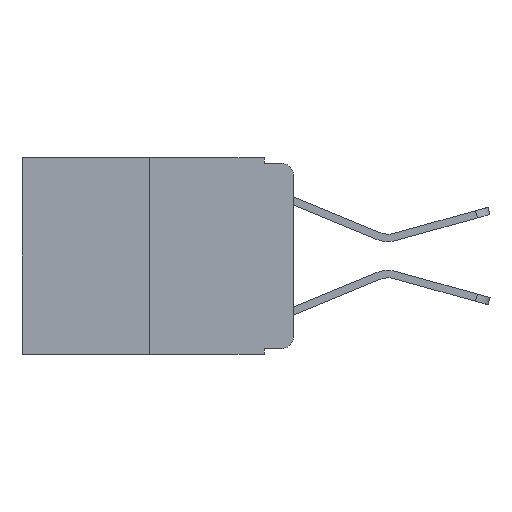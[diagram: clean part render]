
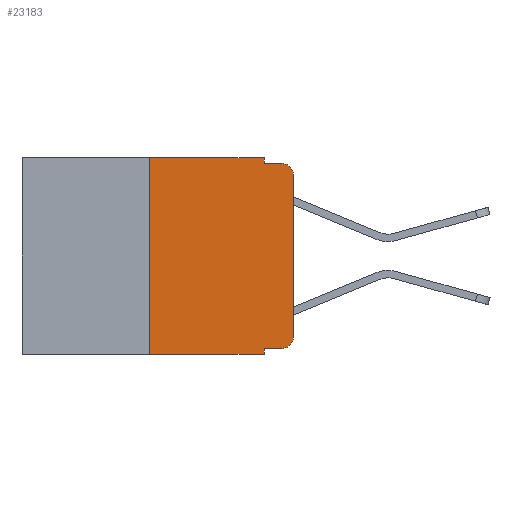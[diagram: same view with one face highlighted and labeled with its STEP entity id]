
A CAD part, left-side view. The second image highlights one B-rep face of the part: STEP entity #23183.
In plain terms, the highlighted planar face has unit normal (-1, 0, 0).
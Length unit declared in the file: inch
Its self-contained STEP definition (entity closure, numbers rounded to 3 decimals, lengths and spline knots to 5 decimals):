
#263 = CARTESIAN_POINT ( 'NONE',  ( 0., 0.473, 0. ) ) ;
#602 = VERTEX_POINT ( 'NONE', #15090 ) ;
#735 = DIRECTION ( 'NONE',  ( 0., 0., -1. ) ) ;
#879 = ORIENTED_EDGE ( 'NONE', *, *, #21196, .T. ) ;
#1485 = CARTESIAN_POINT ( 'NONE',  ( 0., 0.473, -0.343 ) ) ;
#1562 = EDGE_CURVE ( 'NONE', #11115, #17570, #9679, .T. ) ;
#1811 = ORIENTED_EDGE ( 'NONE', *, *, #1562, .T. ) ;
#1951 = ORIENTED_EDGE ( 'NONE', *, *, #12078, .F. ) ;
#2250 = CARTESIAN_POINT ( 'NONE',  ( 0., 0.25, 0. ) ) ;
#3317 = VERTEX_POINT ( 'NONE', #5917 ) ;
#3351 = DIRECTION ( 'NONE',  ( 0., 0., -1. ) ) ;
#3401 = CARTESIAN_POINT ( 'NONE',  ( 0., 0.051, -0.343 ) ) ;
#3549 = EDGE_CURVE ( 'NONE', #8855, #22190, #14930, .T. ) ;
#3611 = CARTESIAN_POINT ( 'NONE',  ( 0., 0., -0.313 ) ) ;
#4162 = CARTESIAN_POINT ( 'NONE',  ( 0., 0.051, -0.01 ) ) ;
#4498 = VECTOR ( 'NONE', #6863, 39.37008 ) ;
#5495 = VERTEX_POINT ( 'NONE', #8070 ) ;
#5668 = DIRECTION ( 'NONE',  ( 0., 0., -1. ) ) ;
#5885 = VERTEX_POINT ( 'NONE', #8922 ) ;
#5917 = CARTESIAN_POINT ( 'NONE',  ( 0., 0.051, -0.333 ) ) ;
#6086 = CARTESIAN_POINT ( 'NONE',  ( 0., 0.02, -0.03 ) ) ;
#6502 = ORIENTED_EDGE ( 'NONE', *, *, #15943, .T. ) ;
#6740 = EDGE_CURVE ( 'NONE', #602, #15473, #20439, .T. ) ;
#6863 = DIRECTION ( 'NONE',  ( 0., 0., 1. ) ) ;
#6919 = VECTOR ( 'NONE', #9512, 39.37008 ) ;
#6938 = VERTEX_POINT ( 'NONE', #21496 ) ;
#8070 = CARTESIAN_POINT ( 'NONE',  ( 0., 0.25, 0. ) ) ;
#8281 = LINE ( 'NONE', #10126, #20691 ) ;
#8409 = ORIENTED_EDGE ( 'NONE', *, *, #22758, .F. ) ;
#8703 = CIRCLE ( 'NONE', #23043, 0.02 ) ;
#8769 = CARTESIAN_POINT ( 'NONE',  ( 0., 0.051, 0. ) ) ;
#8855 = VERTEX_POINT ( 'NONE', #3611 ) ;
#8922 = CARTESIAN_POINT ( 'NONE',  ( 0., 0.02, -0.333 ) ) ;
#9144 = DIRECTION ( 'NONE',  ( 1., 0., 0. ) ) ;
#9228 = EDGE_CURVE ( 'NONE', #5495, #6938, #14072, .T. ) ;
#9345 = ORIENTED_EDGE ( 'NONE', *, *, #3549, .T. ) ;
#9499 = DIRECTION ( 'NONE',  ( 0., 0., 1. ) ) ;
#9512 = DIRECTION ( 'NONE',  ( 0., -1., 0. ) ) ;
#9598 = LINE ( 'NONE', #2250, #11291 ) ;
#9679 = LINE ( 'NONE', #1485, #13357 ) ;
#9899 = DIRECTION ( 'NONE',  ( 0., -1., 0. ) ) ;
#10126 = CARTESIAN_POINT ( 'NONE',  ( 0., 0.051, 0. ) ) ;
#10714 = PLANE ( 'NONE',  #14123 ) ;
#10947 = CARTESIAN_POINT ( 'NONE',  ( 0., 0.25, -0.343 ) ) ;
#11115 = VERTEX_POINT ( 'NONE', #10947 ) ;
#11219 = DIRECTION ( 'NONE',  ( 0., -1., 0. ) ) ;
#11291 = VECTOR ( 'NONE', #9499, 39.37008 ) ;
#11510 = DIRECTION ( 'NONE',  ( -1., 0., 0. ) ) ;
#11651 = CARTESIAN_POINT ( 'NONE',  ( 0., 0.02, -0.01 ) ) ;
#11848 = ORIENTED_EDGE ( 'NONE', *, *, #13816, .F. ) ;
#11943 = DIRECTION ( 'NONE',  ( 0., 0., -1. ) ) ;
#12078 = EDGE_CURVE ( 'NONE', #3317, #17570, #8281, .T. ) ;
#12957 = ORIENTED_EDGE ( 'NONE', *, *, #9228, .F. ) ;
#13031 = LINE ( 'NONE', #16780, #19215 ) ;
#13125 = ORIENTED_EDGE ( 'NONE', *, *, #17053, .T. ) ;
#13357 = VECTOR ( 'NONE', #23028, 39.37008 ) ;
#13458 = LINE ( 'NONE', #8769, #16560 ) ;
#13816 = EDGE_CURVE ( 'NONE', #11115, #5495, #9598, .T. ) ;
#14063 = CIRCLE ( 'NONE', #14606, 0.02 ) ;
#14072 = LINE ( 'NONE', #18905, #23124 ) ;
#14123 = AXIS2_PLACEMENT_3D ( 'NONE', #263, #9144, #5668 ) ;
#14606 = AXIS2_PLACEMENT_3D ( 'NONE', #6086, #11510, #735 ) ;
#14930 = LINE ( 'NONE', #17394, #4498 ) ;
#15090 = CARTESIAN_POINT ( 'NONE',  ( 0., 0.051, -0.01 ) ) ;
#15473 = VERTEX_POINT ( 'NONE', #11651 ) ;
#15943 = EDGE_CURVE ( 'NONE', #3317, #5885, #13031, .T. ) ;
#16034 = DIRECTION ( 'NONE',  ( 0., 0., -1. ) ) ;
#16560 = VECTOR ( 'NONE', #16034, 39.37008 ) ;
#16780 = CARTESIAN_POINT ( 'NONE',  ( 0., 0.051, -0.333 ) ) ;
#17053 = EDGE_CURVE ( 'NONE', #5885, #8855, #8703, .T. ) ;
#17394 = CARTESIAN_POINT ( 'NONE',  ( 0., 0., 0. ) ) ;
#17570 = VERTEX_POINT ( 'NONE', #3401 ) ;
#17814 = EDGE_LOOP ( 'NONE', ( #9345, #879, #21139, #8409, #12957, #11848, #1811, #1951, #6502, #13125 ) ) ;
#17955 = FACE_OUTER_BOUND ( 'NONE', #17814, .T. ) ;
#17976 = CARTESIAN_POINT ( 'NONE',  ( 0., 0., -0.03 ) ) ;
#17977 = DIRECTION ( 'NONE',  ( -1., 0., 0. ) ) ;
#18905 = CARTESIAN_POINT ( 'NONE',  ( 0., 0.473, 0. ) ) ;
#19215 = VECTOR ( 'NONE', #11219, 39.37008 ) ;
#20439 = LINE ( 'NONE', #4162, #6919 ) ;
#20691 = VECTOR ( 'NONE', #11943, 39.37008 ) ;
#21139 = ORIENTED_EDGE ( 'NONE', *, *, #6740, .F. ) ;
#21196 = EDGE_CURVE ( 'NONE', #22190, #15473, #14063, .T. ) ;
#21340 = CARTESIAN_POINT ( 'NONE',  ( 0., 0.02, -0.313 ) ) ;
#21496 = CARTESIAN_POINT ( 'NONE',  ( 0., 0.051, 0. ) ) ;
#22190 = VERTEX_POINT ( 'NONE', #17976 ) ;
#22758 = EDGE_CURVE ( 'NONE', #6938, #602, #13458, .T. ) ;
#23028 = DIRECTION ( 'NONE',  ( 0., -1., 0. ) ) ;
#23043 = AXIS2_PLACEMENT_3D ( 'NONE', #21340, #17977, #3351 ) ;
#23124 = VECTOR ( 'NONE', #9899, 39.37008 ) ;
#23183 = ADVANCED_FACE ( 'NONE', ( #17955 ), #10714, .F. ) ;
